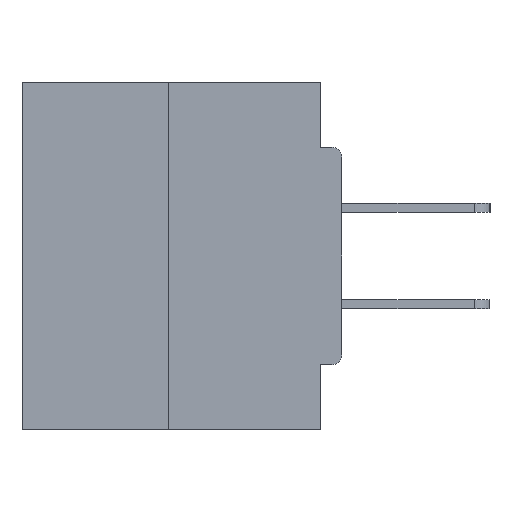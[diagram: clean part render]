
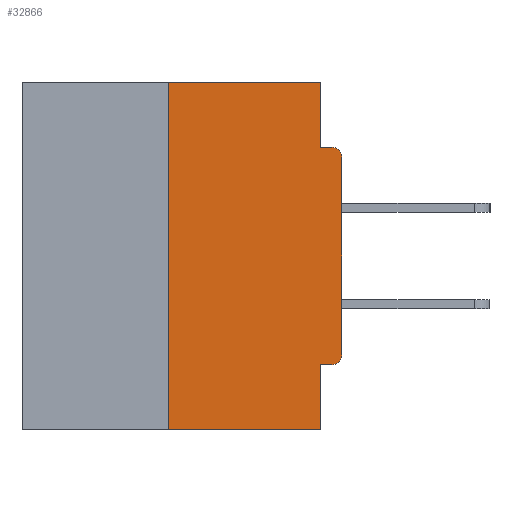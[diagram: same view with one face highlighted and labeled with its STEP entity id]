
A CAD part, left-side view. The second image highlights one B-rep face of the part: STEP entity #32866.
In plain terms, the highlighted planar face has unit normal (-1, 0, 0).
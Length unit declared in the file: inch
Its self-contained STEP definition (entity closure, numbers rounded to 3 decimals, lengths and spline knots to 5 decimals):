
#2006 = VERTEX_POINT ( 'NONE', #21116 ) ;
#3093 = EDGE_CURVE ( 'NONE', #14787, #15675, #35101, .T. ) ;
#3932 = VECTOR ( 'NONE', #9512, 39.37008 ) ;
#4140 = VERTEX_POINT ( 'NONE', #31902 ) ;
#4617 = EDGE_CURVE ( 'NONE', #15675, #12495, #7127, .T. ) ;
#4777 = CARTESIAN_POINT ( 'NONE',  ( 0., 0.25, 0. ) ) ;
#5586 = CARTESIAN_POINT ( 'NONE',  ( 0., 0.46, 0. ) ) ;
#6646 = CARTESIAN_POINT ( 'NONE',  ( 0., 0.015, -0.0935 ) ) ;
#6723 = VECTOR ( 'NONE', #37391, 39.37008 ) ;
#7127 = LINE ( 'NONE', #12453, #3932 ) ;
#7236 = EDGE_CURVE ( 'NONE', #24023, #12495, #33570, .T. ) ;
#7393 = CARTESIAN_POINT ( 'NONE',  ( 0., 0.25, -0.5 ) ) ;
#7511 = CARTESIAN_POINT ( 'NONE',  ( 0., 0.46, -0.5 ) ) ;
#8409 = PLANE ( 'NONE',  #17681 ) ;
#8526 = ORIENTED_EDGE ( 'NONE', *, *, #7236, .T. ) ;
#8672 = CARTESIAN_POINT ( 'NONE',  ( 0., 0.015, -0.3915 ) ) ;
#8796 = DIRECTION ( 'NONE',  ( 0., 0., -1. ) ) ;
#9248 = EDGE_CURVE ( 'NONE', #27753, #22459, #30211, .T. ) ;
#9499 = ORIENTED_EDGE ( 'NONE', *, *, #15347, .T. ) ;
#9512 = DIRECTION ( 'NONE',  ( 0., 0., -1. ) ) ;
#10276 = ORIENTED_EDGE ( 'NONE', *, *, #29216, .T. ) ;
#10459 = CARTESIAN_POINT ( 'NONE',  ( 0., 0.46, 0. ) ) ;
#11263 = ORIENTED_EDGE ( 'NONE', *, *, #3093, .F. ) ;
#11373 = DIRECTION ( 'NONE',  ( 1., 0., 0. ) ) ;
#11759 = ORIENTED_EDGE ( 'NONE', *, *, #27744, .F. ) ;
#12237 = VERTEX_POINT ( 'NONE', #6646 ) ;
#12453 = CARTESIAN_POINT ( 'NONE',  ( 0., 0.031, -0.5 ) ) ;
#12495 = VERTEX_POINT ( 'NONE', #37174 ) ;
#12993 = VECTOR ( 'NONE', #26442, 39.37008 ) ;
#13268 = CARTESIAN_POINT ( 'NONE',  ( 0., 0., -0.0935 ) ) ;
#13395 = DIRECTION ( 'NONE',  ( 0., -1., 0. ) ) ;
#13579 = VECTOR ( 'NONE', #36663, 39.37008 ) ;
#14027 = LINE ( 'NONE', #13268, #13579 ) ;
#14693 = VECTOR ( 'NONE', #31186, 39.37008 ) ;
#14717 = CARTESIAN_POINT ( 'NONE',  ( 0., 0., -0.4065 ) ) ;
#14787 = VERTEX_POINT ( 'NONE', #32500 ) ;
#15347 = EDGE_CURVE ( 'NONE', #14787, #31895, #21773, .T. ) ;
#15529 = DIRECTION ( 'NONE',  ( 0., 0., -1. ) ) ;
#15675 = VERTEX_POINT ( 'NONE', #36879 ) ;
#17681 = AXIS2_PLACEMENT_3D ( 'NONE', #5586, #11373, #8796 ) ;
#18932 = AXIS2_PLACEMENT_3D ( 'NONE', #8672, #23388, #35146 ) ;
#20527 = ORIENTED_EDGE ( 'NONE', *, *, #24356, .F. ) ;
#20657 = EDGE_CURVE ( 'NONE', #2006, #12237, #14027, .T. ) ;
#21116 = CARTESIAN_POINT ( 'NONE',  ( 0., 0.031, -0.0935 ) ) ;
#21162 = CARTESIAN_POINT ( 'NONE',  ( 0., 0.031, 0. ) ) ;
#21773 = CIRCLE ( 'NONE', #18932, 0.015 ) ;
#22051 = CIRCLE ( 'NONE', #37811, 0.015 ) ;
#22459 = VERTEX_POINT ( 'NONE', #21162 ) ;
#23388 = DIRECTION ( 'NONE',  ( -1., 0., 0. ) ) ;
#24023 = VERTEX_POINT ( 'NONE', #7393 ) ;
#24215 = ORIENTED_EDGE ( 'NONE', *, *, #4617, .F. ) ;
#24242 = FACE_OUTER_BOUND ( 'NONE', #36455, .T. ) ;
#24356 = EDGE_CURVE ( 'NONE', #22459, #2006, #37842, .T. ) ;
#25251 = CARTESIAN_POINT ( 'NONE',  ( 0., 0.25, 0. ) ) ;
#25768 = CARTESIAN_POINT ( 'NONE',  ( 0., 0., -0.3915 ) ) ;
#26061 = CARTESIAN_POINT ( 'NONE',  ( 0., 0., 0. ) ) ;
#26442 = DIRECTION ( 'NONE',  ( 0., 0., 1. ) ) ;
#26682 = VECTOR ( 'NONE', #36682, 39.37008 ) ;
#27314 = CARTESIAN_POINT ( 'NONE',  ( 0., 0.015, -0.1085 ) ) ;
#27744 = EDGE_CURVE ( 'NONE', #24023, #27753, #37076, .T. ) ;
#27753 = VERTEX_POINT ( 'NONE', #25251 ) ;
#28777 = CARTESIAN_POINT ( 'NONE',  ( 0., 0.031, 0. ) ) ;
#29216 = EDGE_CURVE ( 'NONE', #31895, #4140, #37675, .T. ) ;
#30211 = LINE ( 'NONE', #10459, #32045 ) ;
#31186 = DIRECTION ( 'NONE',  ( 0., 0., 1. ) ) ;
#31460 = VECTOR ( 'NONE', #35188, 39.37008 ) ;
#31895 = VERTEX_POINT ( 'NONE', #25768 ) ;
#31902 = CARTESIAN_POINT ( 'NONE',  ( 0., 0., -0.1085 ) ) ;
#32045 = VECTOR ( 'NONE', #13395, 39.37008 ) ;
#32500 = CARTESIAN_POINT ( 'NONE',  ( 0., 0.015, -0.4065 ) ) ;
#32866 = ADVANCED_FACE ( 'NONE', ( #24242 ), #8409, .F. ) ;
#33334 = DIRECTION ( 'NONE',  ( -1., 0., 0. ) ) ;
#33570 = LINE ( 'NONE', #7511, #26682 ) ;
#33710 = ORIENTED_EDGE ( 'NONE', *, *, #9248, .F. ) ;
#33975 = ORIENTED_EDGE ( 'NONE', *, *, #35289, .T. ) ;
#34524 = ORIENTED_EDGE ( 'NONE', *, *, #20657, .F. ) ;
#35101 = LINE ( 'NONE', #14717, #31460 ) ;
#35146 = DIRECTION ( 'NONE',  ( 0., 0., -1. ) ) ;
#35188 = DIRECTION ( 'NONE',  ( 0., 1., 0. ) ) ;
#35289 = EDGE_CURVE ( 'NONE', #4140, #12237, #22051, .T. ) ;
#36455 = EDGE_LOOP ( 'NONE', ( #33710, #11759, #8526, #24215, #11263, #9499, #10276, #33975, #34524, #20527 ) ) ;
#36663 = DIRECTION ( 'NONE',  ( 0., -1., 0. ) ) ;
#36682 = DIRECTION ( 'NONE',  ( 0., -1., 0. ) ) ;
#36879 = CARTESIAN_POINT ( 'NONE',  ( 0., 0.031, -0.4065 ) ) ;
#37076 = LINE ( 'NONE', #4777, #14693 ) ;
#37174 = CARTESIAN_POINT ( 'NONE',  ( 0., 0.031, -0.5 ) ) ;
#37391 = DIRECTION ( 'NONE',  ( 0., 0., -1. ) ) ;
#37675 = LINE ( 'NONE', #26061, #12993 ) ;
#37811 = AXIS2_PLACEMENT_3D ( 'NONE', #27314, #33334, #15529 ) ;
#37842 = LINE ( 'NONE', #28777, #6723 ) ;
